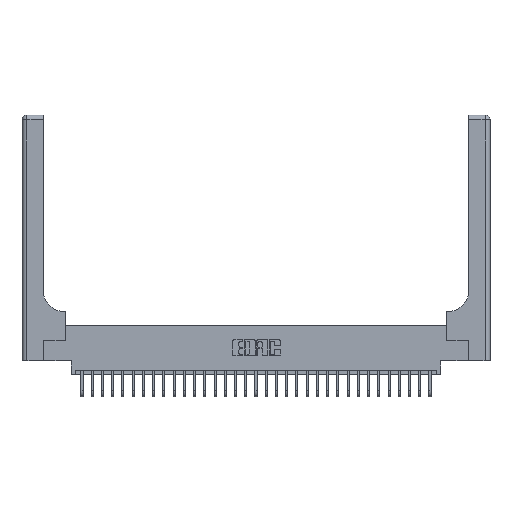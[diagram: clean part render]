
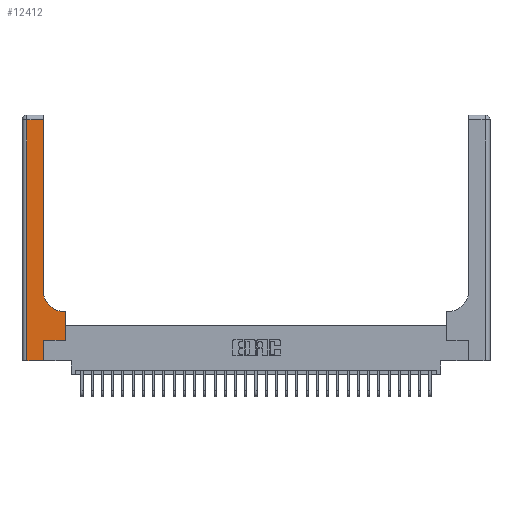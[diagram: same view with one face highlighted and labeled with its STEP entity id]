
A CAD part, top view. The second image highlights one B-rep face of the part: STEP entity #12412.
In plain terms, the highlighted planar face has unit normal (0, 0, 1).
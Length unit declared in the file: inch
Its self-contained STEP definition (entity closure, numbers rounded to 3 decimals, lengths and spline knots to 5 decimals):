
#963 = ORIENTED_EDGE ( 'NONE', *, *, #21907, .T. ) ;
#1181 = DIRECTION ( 'NONE',  ( 0., 1., 0. ) ) ;
#1504 = DIRECTION ( 'NONE',  ( 1., 0., 0. ) ) ;
#2138 = EDGE_CURVE ( 'NONE', #2535, #29431, #29169, .T. ) ;
#2163 = DIRECTION ( 'NONE',  ( 0., 0., -1. ) ) ;
#2535 = VERTEX_POINT ( 'NONE', #7836 ) ;
#2607 = VERTEX_POINT ( 'NONE', #26860 ) ;
#4624 = EDGE_CURVE ( 'NONE', #2607, #24955, #15316, .T. ) ;
#4628 = ORIENTED_EDGE ( 'NONE', *, *, #22102, .T. ) ;
#4714 = DIRECTION ( 'NONE',  ( -1., 0., 0. ) ) ;
#5599 = LINE ( 'NONE', #22765, #9311 ) ;
#6009 = CARTESIAN_POINT ( 'NONE',  ( 0.528, 0.25, 0.37 ) ) ;
#6845 = VECTOR ( 'NONE', #15280, 39.37008 ) ;
#7234 = ORIENTED_EDGE ( 'NONE', *, *, #12995, .T. ) ;
#7269 = LINE ( 'NONE', #19188, #10992 ) ;
#7555 = EDGE_CURVE ( 'NONE', #13143, #11640, #29699, .T. ) ;
#7752 = VERTEX_POINT ( 'NONE', #9237 ) ;
#7836 = CARTESIAN_POINT ( 'NONE',  ( 0.06, 0., 0.37 ) ) ;
#8034 = ORIENTED_EDGE ( 'NONE', *, *, #20288, .T. ) ;
#8758 = CARTESIAN_POINT ( 'NONE',  ( 0.06, 3., 0.37 ) ) ;
#8956 = CARTESIAN_POINT ( 'NONE',  ( 0.265, 0.25, 0.37 ) ) ;
#9237 = CARTESIAN_POINT ( 'NONE',  ( 0.51, 0.6, 0.37 ) ) ;
#9311 = VECTOR ( 'NONE', #15318, 39.37008 ) ;
#9373 = FACE_OUTER_BOUND ( 'NONE', #15693, .T. ) ;
#9542 = PLANE ( 'NONE',  #10821 ) ;
#10532 = CARTESIAN_POINT ( 'NONE',  ( 0.265, 0.25, 0.37 ) ) ;
#10821 = AXIS2_PLACEMENT_3D ( 'NONE', #14621, #2163, #4714 ) ;
#10843 = LINE ( 'NONE', #8758, #22120 ) ;
#10992 = VECTOR ( 'NONE', #16950, 39.37008 ) ;
#11423 = CARTESIAN_POINT ( 'NONE',  ( 0.51, 0.85, 0.37 ) ) ;
#11640 = VERTEX_POINT ( 'NONE', #23870 ) ;
#12412 = ADVANCED_FACE ( 'NONE', ( #9373 ), #9542, .F. ) ;
#12995 = EDGE_CURVE ( 'NONE', #24556, #7752, #5599, .T. ) ;
#13081 = CARTESIAN_POINT ( 'NONE',  ( 0.06, 2.94, 0.37 ) ) ;
#13143 = VERTEX_POINT ( 'NONE', #8956 ) ;
#13173 = VECTOR ( 'NONE', #22419, 39.37008 ) ;
#13331 = ORIENTED_EDGE ( 'NONE', *, *, #15392, .T. ) ;
#14439 = ORIENTED_EDGE ( 'NONE', *, *, #7555, .T. ) ;
#14613 = CARTESIAN_POINT ( 'NONE',  ( 0., 0., 0.37 ) ) ;
#14621 = CARTESIAN_POINT ( 'NONE',  ( 0., 3., 0.37 ) ) ;
#15280 = DIRECTION ( 'NONE',  ( -1., 0., 0. ) ) ;
#15316 = LINE ( 'NONE', #29885, #18046 ) ;
#15318 = DIRECTION ( 'NONE',  ( -1., 0., 0. ) ) ;
#15392 = EDGE_CURVE ( 'NONE', #11640, #24556, #22985, .T. ) ;
#15693 = EDGE_LOOP ( 'NONE', ( #26773, #8034, #963, #24763, #4628, #14439, #13331, #7234, #20280 ) ) ;
#16950 = DIRECTION ( 'NONE',  ( 0., 1., 0. ) ) ;
#17661 = AXIS2_PLACEMENT_3D ( 'NONE', #11423, #30417, #1504 ) ;
#17947 = LINE ( 'NONE', #30149, #6845 ) ;
#17948 = CARTESIAN_POINT ( 'NONE',  ( 0.26, 2.94, 0.37 ) ) ;
#18046 = VECTOR ( 'NONE', #24660, 39.37008 ) ;
#18281 = DIRECTION ( 'NONE',  ( 0., -1., 0. ) ) ;
#19188 = CARTESIAN_POINT ( 'NONE',  ( 0.265, 0., 0.37 ) ) ;
#19490 = EDGE_CURVE ( 'NONE', #7752, #2607, #27273, .T. ) ;
#19580 = VECTOR ( 'NONE', #1181, 39.37008 ) ;
#20280 = ORIENTED_EDGE ( 'NONE', *, *, #19490, .T. ) ;
#20288 = EDGE_CURVE ( 'NONE', #24955, #28393, #17947, .T. ) ;
#21907 = EDGE_CURVE ( 'NONE', #28393, #2535, #10843, .T. ) ;
#22102 = EDGE_CURVE ( 'NONE', #29431, #13143, #7269, .T. ) ;
#22109 = CARTESIAN_POINT ( 'NONE',  ( 0.265, 0., 0.37 ) ) ;
#22120 = VECTOR ( 'NONE', #18281, 39.37008 ) ;
#22419 = DIRECTION ( 'NONE',  ( 1., 0., 0. ) ) ;
#22765 = CARTESIAN_POINT ( 'NONE',  ( 0.26, 0.6, 0.37 ) ) ;
#22985 = LINE ( 'NONE', #6009, #19580 ) ;
#23870 = CARTESIAN_POINT ( 'NONE',  ( 0.528, 0.25, 0.37 ) ) ;
#24556 = VERTEX_POINT ( 'NONE', #25600 ) ;
#24660 = DIRECTION ( 'NONE',  ( 0., 1., 0. ) ) ;
#24763 = ORIENTED_EDGE ( 'NONE', *, *, #2138, .T. ) ;
#24955 = VERTEX_POINT ( 'NONE', #17948 ) ;
#25600 = CARTESIAN_POINT ( 'NONE',  ( 0.528, 0.6, 0.37 ) ) ;
#26773 = ORIENTED_EDGE ( 'NONE', *, *, #4624, .T. ) ;
#26785 = DIRECTION ( 'NONE',  ( 1., 0., 0. ) ) ;
#26860 = CARTESIAN_POINT ( 'NONE',  ( 0.26, 0.85, 0.37 ) ) ;
#27273 = CIRCLE ( 'NONE', #17661, 0.25 ) ;
#28393 = VERTEX_POINT ( 'NONE', #13081 ) ;
#29169 = LINE ( 'NONE', #14613, #30653 ) ;
#29431 = VERTEX_POINT ( 'NONE', #22109 ) ;
#29699 = LINE ( 'NONE', #10532, #13173 ) ;
#29885 = CARTESIAN_POINT ( 'NONE',  ( 0.26, 3., 0.37 ) ) ;
#30149 = CARTESIAN_POINT ( 'NONE',  ( 0., 2.94, 0.37 ) ) ;
#30417 = DIRECTION ( 'NONE',  ( 0., 0., -1. ) ) ;
#30653 = VECTOR ( 'NONE', #26785, 39.37008 ) ;
